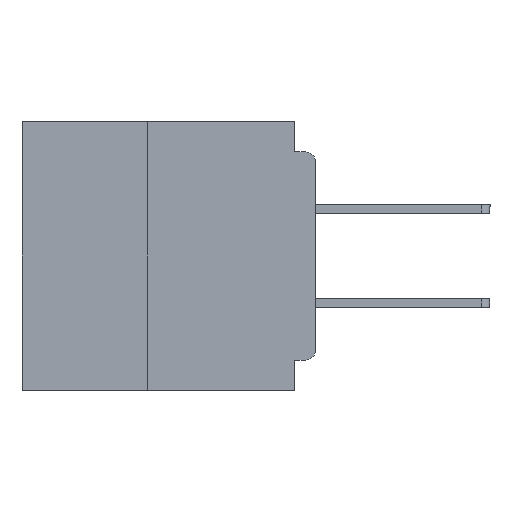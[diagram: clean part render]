
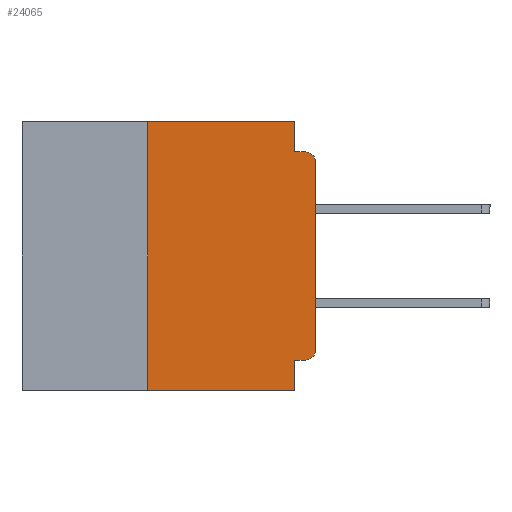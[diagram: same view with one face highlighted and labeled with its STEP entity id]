
A CAD part, left-side view. The second image highlights one B-rep face of the part: STEP entity #24065.
In plain terms, the highlighted planar face has unit normal (-1, 0, 0).
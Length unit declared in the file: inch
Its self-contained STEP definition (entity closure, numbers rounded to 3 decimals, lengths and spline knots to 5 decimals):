
#221 = CARTESIAN_POINT ( 'NONE',  ( 0., 0.015, -0.06 ) ) ;
#580 = EDGE_CURVE ( 'NONE', #30437, #23778, #7929, .T. ) ;
#637 = DIRECTION ( 'NONE',  ( 0., 0., 1. ) ) ;
#1742 = CARTESIAN_POINT ( 'NONE',  ( 0., 0.437, 0. ) ) ;
#2149 = CARTESIAN_POINT ( 'NONE',  ( 0., 0.015, -0.355 ) ) ;
#2735 = VECTOR ( 'NONE', #5181, 39.37008 ) ;
#2772 = CARTESIAN_POINT ( 'NONE',  ( 0., 0., -0.06 ) ) ;
#3468 = AXIS2_PLACEMENT_3D ( 'NONE', #221, #25453, #3846 ) ;
#3493 = CARTESIAN_POINT ( 'NONE',  ( 0., 0.031, -0.4 ) ) ;
#3815 = CARTESIAN_POINT ( 'NONE',  ( 0., 0.031, -0.4 ) ) ;
#3846 = DIRECTION ( 'NONE',  ( 0., 0., -1. ) ) ;
#4018 = CIRCLE ( 'NONE', #9995, 0.015 ) ;
#5181 = DIRECTION ( 'NONE',  ( 0., -1., 0. ) ) ;
#5387 = DIRECTION ( 'NONE',  ( 0., 0., -1. ) ) ;
#5436 = EDGE_CURVE ( 'NONE', #29031, #23778, #27568, .T. ) ;
#6205 = CARTESIAN_POINT ( 'NONE',  ( 0., 0., -0.355 ) ) ;
#6720 = CARTESIAN_POINT ( 'NONE',  ( 0., 0.25, -0.4 ) ) ;
#7198 = CARTESIAN_POINT ( 'NONE',  ( 0., 0., -0.34 ) ) ;
#7531 = ORIENTED_EDGE ( 'NONE', *, *, #580, .F. ) ;
#7929 = LINE ( 'NONE', #3815, #45363 ) ;
#9482 = CARTESIAN_POINT ( 'NONE',  ( 0., 0.031, 0. ) ) ;
#9612 = VECTOR ( 'NONE', #34888, 39.37008 ) ;
#9995 = AXIS2_PLACEMENT_3D ( 'NONE', #17834, #43243, #21486 ) ;
#10252 = EDGE_CURVE ( 'NONE', #29031, #12875, #15404, .T. ) ;
#10872 = VECTOR ( 'NONE', #27971, 39.37008 ) ;
#10892 = EDGE_LOOP ( 'NONE', ( #16537, #37063, #18830, #28417, #11442, #12580, #34185, #7531, #30167, #12030 ) ) ;
#11196 = VERTEX_POINT ( 'NONE', #7198 ) ;
#11291 = CARTESIAN_POINT ( 'NONE',  ( 0., 0.031, 0. ) ) ;
#11442 = ORIENTED_EDGE ( 'NONE', *, *, #18598, .F. ) ;
#11996 = LINE ( 'NONE', #6205, #10872 ) ;
#12030 = ORIENTED_EDGE ( 'NONE', *, *, #46174, .T. ) ;
#12580 = ORIENTED_EDGE ( 'NONE', *, *, #10252, .F. ) ;
#12817 = CARTESIAN_POINT ( 'NONE',  ( 0., 0.25, -0.4 ) ) ;
#12875 = VERTEX_POINT ( 'NONE', #39281 ) ;
#14397 = CARTESIAN_POINT ( 'NONE',  ( 0., 0.015, -0.045 ) ) ;
#14448 = CARTESIAN_POINT ( 'NONE',  ( 0., 0.031, -0.355 ) ) ;
#15177 = CARTESIAN_POINT ( 'NONE',  ( 0., 0., -0.045 ) ) ;
#15404 = LINE ( 'NONE', #12817, #33585 ) ;
#16469 = DIRECTION ( 'NONE',  ( 0., 0., 1. ) ) ;
#16537 = ORIENTED_EDGE ( 'NONE', *, *, #16673, .T. ) ;
#16673 = EDGE_CURVE ( 'NONE', #11196, #18833, #46022, .T. ) ;
#17484 = EDGE_CURVE ( 'NONE', #36464, #46147, #19244, .T. ) ;
#17834 = CARTESIAN_POINT ( 'NONE',  ( 0., 0.015, -0.34 ) ) ;
#18598 = EDGE_CURVE ( 'NONE', #12875, #36464, #32729, .T. ) ;
#18830 = ORIENTED_EDGE ( 'NONE', *, *, #27265, .F. ) ;
#18833 = VERTEX_POINT ( 'NONE', #2772 ) ;
#19244 = LINE ( 'NONE', #9482, #9612 ) ;
#19560 = DIRECTION ( 'NONE',  ( 0., 0., -1. ) ) ;
#21486 = DIRECTION ( 'NONE',  ( 0., 0., -1. ) ) ;
#22249 = CARTESIAN_POINT ( 'NONE',  ( 0., 0., 0. ) ) ;
#22463 = DIRECTION ( 'NONE',  ( 0., -1., 0. ) ) ;
#23343 = EDGE_CURVE ( 'NONE', #18833, #35061, #30866, .T. ) ;
#23778 = VERTEX_POINT ( 'NONE', #3493 ) ;
#24065 = ADVANCED_FACE ( 'NONE', ( #36024 ), #41512, .F. ) ;
#25453 = DIRECTION ( 'NONE',  ( -1., 0., 0. ) ) ;
#26430 = VECTOR ( 'NONE', #40578, 39.37008 ) ;
#27004 = DIRECTION ( 'NONE',  ( 1., 0., 0. ) ) ;
#27265 = EDGE_CURVE ( 'NONE', #46147, #35061, #45591, .T. ) ;
#27407 = AXIS2_PLACEMENT_3D ( 'NONE', #1742, #27004, #5387 ) ;
#27568 = LINE ( 'NONE', #36968, #26430 ) ;
#27971 = DIRECTION ( 'NONE',  ( 0., 1., 0. ) ) ;
#28417 = ORIENTED_EDGE ( 'NONE', *, *, #17484, .F. ) ;
#29031 = VERTEX_POINT ( 'NONE', #6720 ) ;
#30167 = ORIENTED_EDGE ( 'NONE', *, *, #35561, .F. ) ;
#30437 = VERTEX_POINT ( 'NONE', #14448 ) ;
#30866 = CIRCLE ( 'NONE', #3468, 0.015 ) ;
#32729 = LINE ( 'NONE', #37848, #2735 ) ;
#33585 = VECTOR ( 'NONE', #16469, 39.37008 ) ;
#34185 = ORIENTED_EDGE ( 'NONE', *, *, #5436, .T. ) ;
#34781 = VERTEX_POINT ( 'NONE', #2149 ) ;
#34888 = DIRECTION ( 'NONE',  ( 0., 0., -1. ) ) ;
#35061 = VERTEX_POINT ( 'NONE', #14397 ) ;
#35561 = EDGE_CURVE ( 'NONE', #34781, #30437, #11996, .T. ) ;
#35678 = CARTESIAN_POINT ( 'NONE',  ( 0., 0.031, -0.045 ) ) ;
#35962 = VECTOR ( 'NONE', #22463, 39.37008 ) ;
#36024 = FACE_OUTER_BOUND ( 'NONE', #10892, .T. ) ;
#36395 = VECTOR ( 'NONE', #637, 39.37008 ) ;
#36464 = VERTEX_POINT ( 'NONE', #11291 ) ;
#36968 = CARTESIAN_POINT ( 'NONE',  ( 0., 0.437, -0.4 ) ) ;
#37063 = ORIENTED_EDGE ( 'NONE', *, *, #23343, .T. ) ;
#37848 = CARTESIAN_POINT ( 'NONE',  ( 0., 0.437, 0. ) ) ;
#39281 = CARTESIAN_POINT ( 'NONE',  ( 0., 0.25, 0. ) ) ;
#40578 = DIRECTION ( 'NONE',  ( 0., -1., 0. ) ) ;
#41512 = PLANE ( 'NONE',  #27407 ) ;
#43243 = DIRECTION ( 'NONE',  ( -1., 0., 0. ) ) ;
#45363 = VECTOR ( 'NONE', #19560, 39.37008 ) ;
#45591 = LINE ( 'NONE', #15177, #35962 ) ;
#46022 = LINE ( 'NONE', #22249, #36395 ) ;
#46147 = VERTEX_POINT ( 'NONE', #35678 ) ;
#46174 = EDGE_CURVE ( 'NONE', #34781, #11196, #4018, .T. ) ;
